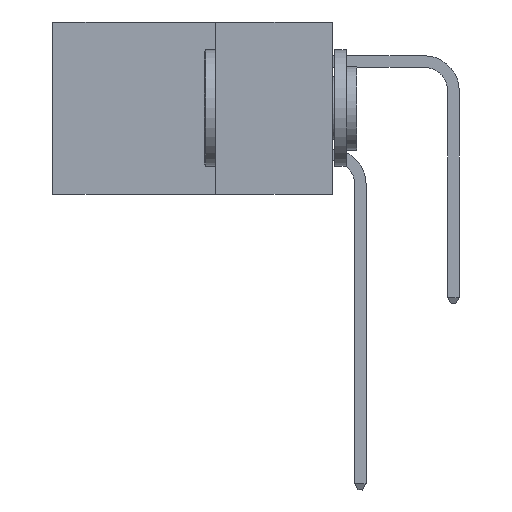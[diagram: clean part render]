
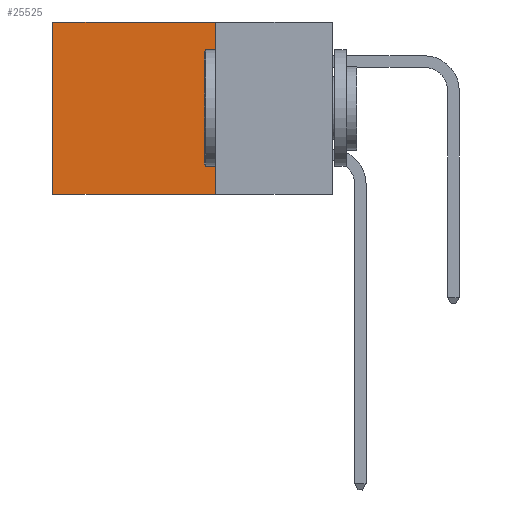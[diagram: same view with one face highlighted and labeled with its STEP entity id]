
A CAD part, left-side view. The second image highlights one B-rep face of the part: STEP entity #25525.
In plain terms, the highlighted planar face has unit normal (-1, 0, 0).
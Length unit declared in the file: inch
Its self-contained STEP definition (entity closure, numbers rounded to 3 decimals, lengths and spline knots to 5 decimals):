
#565 = EDGE_CURVE ( 'NONE', #2528, #18265, #23060, .T. ) ;
#1041 = DIRECTION ( 'NONE',  ( 0., 0., -1. ) ) ;
#1502 = VECTOR ( 'NONE', #8903, 39.37008 ) ;
#1709 = EDGE_CURVE ( 'NONE', #2528, #5142, #23651, .T. ) ;
#2071 = EDGE_LOOP ( 'NONE', ( #21234, #9563, #6938, #21560 ) ) ;
#2496 = VECTOR ( 'NONE', #1041, 39.37008 ) ;
#2528 = VERTEX_POINT ( 'NONE', #16384 ) ;
#4181 = CARTESIAN_POINT ( 'NONE',  ( 0.298, 0.25, -0.37 ) ) ;
#4813 = PLANE ( 'NONE',  #10945 ) ;
#4887 = CARTESIAN_POINT ( 'NONE',  ( 0.298, 0.25, -0.37 ) ) ;
#5142 = VERTEX_POINT ( 'NONE', #12310 ) ;
#6841 = CARTESIAN_POINT ( 'NONE',  ( 0.298, 0.25, 0. ) ) ;
#6938 = ORIENTED_EDGE ( 'NONE', *, *, #565, .F. ) ;
#6968 = LINE ( 'NONE', #4181, #1502 ) ;
#7385 = LINE ( 'NONE', #12299, #21508 ) ;
#8903 = DIRECTION ( 'NONE',  ( 0., 1., 0. ) ) ;
#9563 = ORIENTED_EDGE ( 'NONE', *, *, #25455, .F. ) ;
#10317 = DIRECTION ( 'NONE',  ( 0., 0., -1. ) ) ;
#10945 = AXIS2_PLACEMENT_3D ( 'NONE', #6841, #14768, #23357 ) ;
#12299 = CARTESIAN_POINT ( 'NONE',  ( 0.298, 0.6, 0. ) ) ;
#12310 = CARTESIAN_POINT ( 'NONE',  ( 0.298, 0.6, 0. ) ) ;
#12669 = CARTESIAN_POINT ( 'NONE',  ( 0.298, 0.25, 0. ) ) ;
#14768 = DIRECTION ( 'NONE',  ( 1., 0., 0. ) ) ;
#16384 = CARTESIAN_POINT ( 'NONE',  ( 0.298, 0.25, 0. ) ) ;
#17854 = CARTESIAN_POINT ( 'NONE',  ( 0.298, 0.25, 0. ) ) ;
#17877 = VERTEX_POINT ( 'NONE', #26427 ) ;
#18265 = VERTEX_POINT ( 'NONE', #4887 ) ;
#19480 = VECTOR ( 'NONE', #25022, 39.37008 ) ;
#21234 = ORIENTED_EDGE ( 'NONE', *, *, #23404, .T. ) ;
#21508 = VECTOR ( 'NONE', #10317, 39.37008 ) ;
#21560 = ORIENTED_EDGE ( 'NONE', *, *, #1709, .T. ) ;
#23060 = LINE ( 'NONE', #17854, #2496 ) ;
#23357 = DIRECTION ( 'NONE',  ( 0., 0., -1. ) ) ;
#23404 = EDGE_CURVE ( 'NONE', #5142, #17877, #7385, .T. ) ;
#23651 = LINE ( 'NONE', #12669, #19480 ) ;
#24942 = FACE_OUTER_BOUND ( 'NONE', #2071, .T. ) ;
#25022 = DIRECTION ( 'NONE',  ( 0., 1., 0. ) ) ;
#25455 = EDGE_CURVE ( 'NONE', #18265, #17877, #6968, .T. ) ;
#25525 = ADVANCED_FACE ( 'NONE', ( #24942 ), #4813, .F. ) ;
#26427 = CARTESIAN_POINT ( 'NONE',  ( 0.298, 0.6, -0.37 ) ) ;
